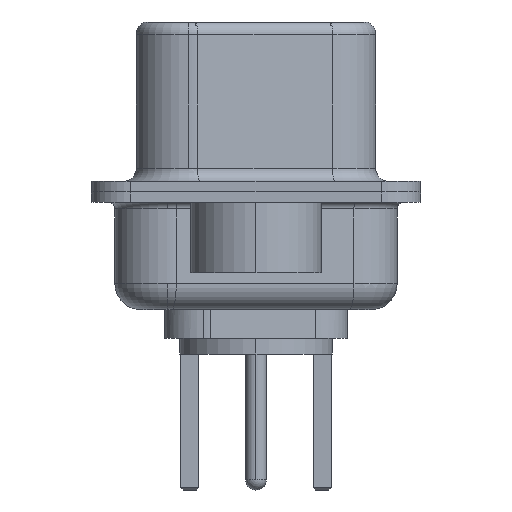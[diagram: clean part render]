
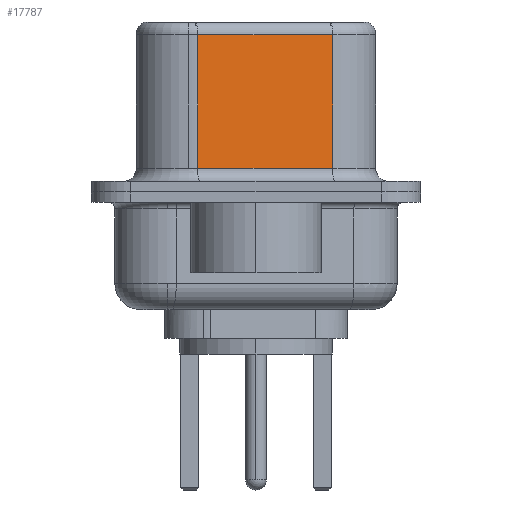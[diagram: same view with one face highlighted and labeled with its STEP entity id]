
A CAD part, left-side view. The second image highlights one B-rep face of the part: STEP entity #17787.
In plain terms, the highlighted planar face has unit normal (-0.985, -0.174, 0).
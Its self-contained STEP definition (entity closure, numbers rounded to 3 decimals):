
#929 = CARTESIAN_POINT ( 'NONE',  ( 4.58, -2.927, 0.9 ) ) ;
#1089 = CARTESIAN_POINT ( 'NONE',  ( 3.67, 2.233, 6.02 ) ) ;
#1125 = EDGE_CURVE ( 'NONE', #7357, #12761, #10807, .T. ) ;
#1280 = EDGE_LOOP ( 'NONE', ( #10434, #9354, #14029, #13640 ) ) ;
#1860 = EDGE_CURVE ( 'NONE', #12761, #15785, #11439, .T. ) ;
#2032 = CARTESIAN_POINT ( 'NONE',  ( 4.58, -2.927, 6.52 ) ) ;
#2246 = CARTESIAN_POINT ( 'NONE',  ( 4.58, -2.927, 6.02 ) ) ;
#2466 = VERTEX_POINT ( 'NONE', #14624 ) ;
#3464 = DIRECTION ( 'NONE',  ( 0.985, 0.174, 0. ) ) ;
#3908 = DIRECTION ( 'NONE',  ( 0., 0., -1. ) ) ;
#5136 = CARTESIAN_POINT ( 'NONE',  ( 4.58, -2.927, 6.52 ) ) ;
#6722 = EDGE_CURVE ( 'NONE', #7357, #2466, #16706, .T. ) ;
#6912 = DIRECTION ( 'NONE',  ( 0., 0., -1. ) ) ;
#7357 = VERTEX_POINT ( 'NONE', #2246 ) ;
#9005 = AXIS2_PLACEMENT_3D ( 'NONE', #2032, #3464, #13551 ) ;
#9354 = ORIENTED_EDGE ( 'NONE', *, *, #1125, .T. ) ;
#9531 = DIRECTION ( 'NONE',  ( 0.174, -0.985, 0. ) ) ;
#10434 = ORIENTED_EDGE ( 'NONE', *, *, #6722, .F. ) ;
#10485 = EDGE_CURVE ( 'NONE', #15785, #2466, #13213, .T. ) ;
#10807 = LINE ( 'NONE', #11630, #13705 ) ;
#11125 = CARTESIAN_POINT ( 'NONE',  ( 3.67, 2.233, 6.52 ) ) ;
#11439 = LINE ( 'NONE', #11125, #12971 ) ;
#11556 = VECTOR ( 'NONE', #3908, 1000. ) ;
#11630 = CARTESIAN_POINT ( 'NONE',  ( 4.58, -2.927, 6.02 ) ) ;
#12761 = VERTEX_POINT ( 'NONE', #1089 ) ;
#12971 = VECTOR ( 'NONE', #6912, 1000. ) ;
#13213 = LINE ( 'NONE', #929, #15911 ) ;
#13551 = DIRECTION ( 'NONE',  ( -0.174, 0.985, 0. ) ) ;
#13640 = ORIENTED_EDGE ( 'NONE', *, *, #10485, .T. ) ;
#13705 = VECTOR ( 'NONE', #14491, 1000. ) ;
#14029 = ORIENTED_EDGE ( 'NONE', *, *, #1860, .T. ) ;
#14491 = DIRECTION ( 'NONE',  ( -0.174, 0.985, 0. ) ) ;
#14624 = CARTESIAN_POINT ( 'NONE',  ( 4.58, -2.927, 0.9 ) ) ;
#14931 = PLANE ( 'NONE',  #9005 ) ;
#15785 = VERTEX_POINT ( 'NONE', #17275 ) ;
#15911 = VECTOR ( 'NONE', #9531, 1000. ) ;
#16417 = FACE_OUTER_BOUND ( 'NONE', #1280, .T. ) ;
#16706 = LINE ( 'NONE', #5136, #11556 ) ;
#17275 = CARTESIAN_POINT ( 'NONE',  ( 3.67, 2.233, 0.9 ) ) ;
#17787 = ADVANCED_FACE ( 'NONE', ( #16417 ), #14931, .F. ) ;
